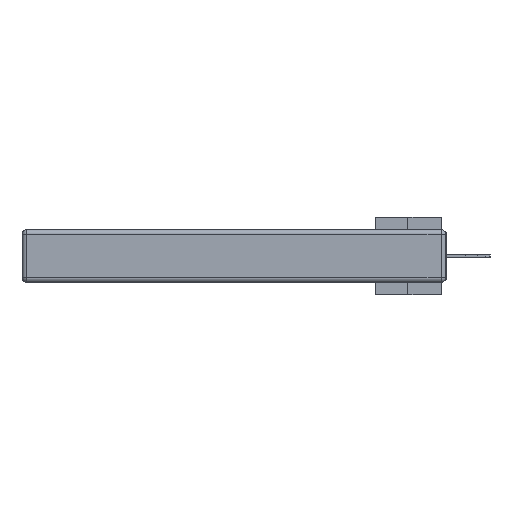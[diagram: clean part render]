
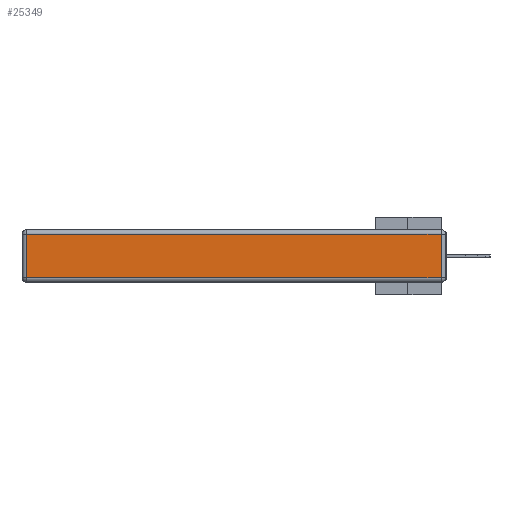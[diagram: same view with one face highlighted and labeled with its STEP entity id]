
A CAD part, left-side view. The second image highlights one B-rep face of the part: STEP entity #25349.
In plain terms, the highlighted planar face has unit normal (-1, 0, 0).
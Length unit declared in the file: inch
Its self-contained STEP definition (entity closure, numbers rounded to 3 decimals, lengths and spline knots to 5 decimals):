
#1634 = DIRECTION ( 'NONE',  ( 0., 0., 1. ) ) ;
#2045 = VERTEX_POINT ( 'NONE', #31810 ) ;
#2077 = CARTESIAN_POINT ( 'NONE',  ( 0., 0.03, -0.343 ) ) ;
#3010 = LINE ( 'NONE', #10255, #5139 ) ;
#3493 = CARTESIAN_POINT ( 'NONE',  ( 0., 2.72, -0.313 ) ) ;
#3630 = CARTESIAN_POINT ( 'NONE',  ( 0., 0.03, -0.03 ) ) ;
#4223 = CARTESIAN_POINT ( 'NONE',  ( 0., 0., -0.313 ) ) ;
#5139 = VECTOR ( 'NONE', #13596, 39.37008 ) ;
#5612 = EDGE_CURVE ( 'NONE', #17675, #42634, #13358, .T. ) ;
#7621 = DIRECTION ( 'NONE',  ( 0., -1., 0. ) ) ;
#9742 = EDGE_CURVE ( 'NONE', #38142, #2045, #14807, .T. ) ;
#10255 = CARTESIAN_POINT ( 'NONE',  ( 0., 2.72, -0.343 ) ) ;
#11424 = FACE_OUTER_BOUND ( 'NONE', #22820, .T. ) ;
#13358 = LINE ( 'NONE', #32130, #28776 ) ;
#13596 = DIRECTION ( 'NONE',  ( 0., 0., -1. ) ) ;
#13765 = VECTOR ( 'NONE', #7621, 39.37008 ) ;
#14807 = LINE ( 'NONE', #4223, #13765 ) ;
#15636 = ORIENTED_EDGE ( 'NONE', *, *, #5612, .T. ) ;
#15820 = DIRECTION ( 'NONE',  ( 0., 1., 0. ) ) ;
#15868 = EDGE_CURVE ( 'NONE', #42634, #38142, #3010, .T. ) ;
#16024 = VECTOR ( 'NONE', #38434, 39.37008 ) ;
#16656 = ORIENTED_EDGE ( 'NONE', *, *, #9742, .T. ) ;
#17675 = VERTEX_POINT ( 'NONE', #3630 ) ;
#20339 = CARTESIAN_POINT ( 'NONE',  ( 0., 2.72, -0.03 ) ) ;
#21636 = DIRECTION ( 'NONE',  ( -1., 0., 0. ) ) ;
#22820 = EDGE_LOOP ( 'NONE', ( #16656, #22883, #15636, #25110 ) ) ;
#22883 = ORIENTED_EDGE ( 'NONE', *, *, #32448, .T. ) ;
#25110 = ORIENTED_EDGE ( 'NONE', *, *, #15868, .T. ) ;
#25349 = ADVANCED_FACE ( 'NONE', ( #11424 ), #37996, .T. ) ;
#28097 = CARTESIAN_POINT ( 'NONE',  ( 0., 0., -0.343 ) ) ;
#28776 = VECTOR ( 'NONE', #15820, 39.37008 ) ;
#31810 = CARTESIAN_POINT ( 'NONE',  ( 0., 0.03, -0.313 ) ) ;
#32130 = CARTESIAN_POINT ( 'NONE',  ( 0., 2.75, -0.03 ) ) ;
#32448 = EDGE_CURVE ( 'NONE', #2045, #17675, #42138, .T. ) ;
#37996 = PLANE ( 'NONE',  #39233 ) ;
#38142 = VERTEX_POINT ( 'NONE', #3493 ) ;
#38434 = DIRECTION ( 'NONE',  ( 0., 0., 1. ) ) ;
#39233 = AXIS2_PLACEMENT_3D ( 'NONE', #28097, #21636, #1634 ) ;
#42138 = LINE ( 'NONE', #2077, #16024 ) ;
#42634 = VERTEX_POINT ( 'NONE', #20339 ) ;
